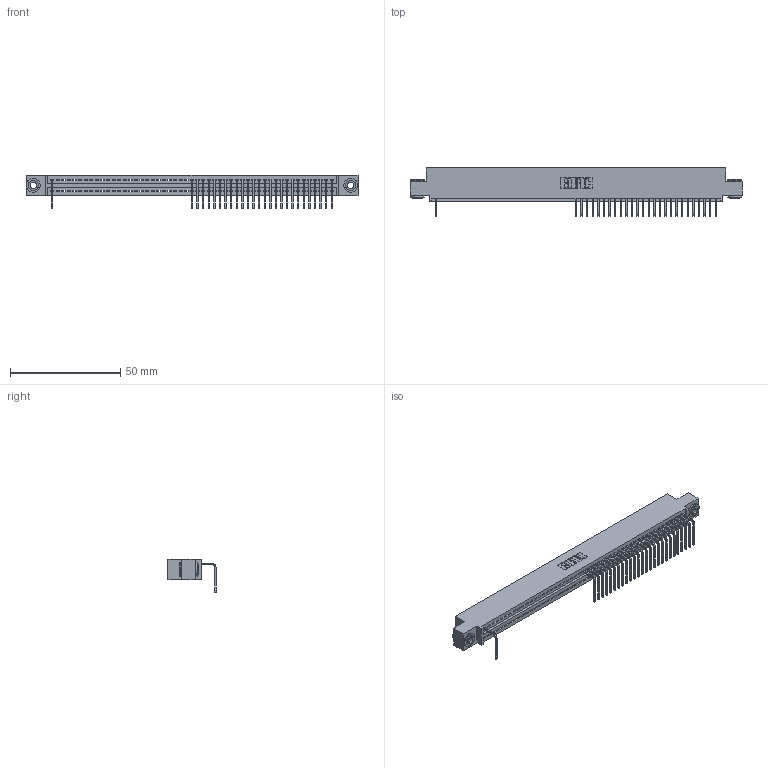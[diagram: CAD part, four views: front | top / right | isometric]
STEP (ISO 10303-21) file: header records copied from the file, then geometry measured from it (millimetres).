
FILE_DESCRIPTION (( 'STEP AP203' ), '1' );
FILE_NAME ('345-051-558-403.STEP', '2018-09-22T18:34:22', ( '' ), ( '' ), 'SwSTEP 2.0', 'SolidWorks 2016', '' );
FILE_SCHEMA (( 'CONFIG_CONTROL_DESIGN' ));
Length unit declared in the file: inch
Products named in the file (4): 345 Part_0.110 Offset - 0.156 Dia-TH; 345-292-001_558 Tail - 2; 345-250-002_345-250-002-102; 345-051-558-403
Assembly tree (30 placements, depth 2):
  345-051-558-403
    345 Part_0.110 Offset - 0.156 Dia-TH
    345-292-001_558 Tail - 2  x27
    345-250-002_345-250-002-102  x2
Bounding box: 150.75 x 21.83 x 15.37 mm (x, y, z)
Volume: 14153.2 mm3; surface area: 18296.2 mm2
Topology: 30 solids, 30 shells, 2172 faces, 6639 edges, 4386 vertices
Faces by surface type: plane 1564, cylinder 600, cone 8
Entity records: 37270 total; most frequent: ORIENTED_EDGE 6546, CARTESIAN_POINT 6544, DIRECTION 5705, EDGE_CURVE 3273, LINE 2913, VECTOR 2913, VERTEX_POINT 2178, AXIS2_PLACEMENT_3D 1396
